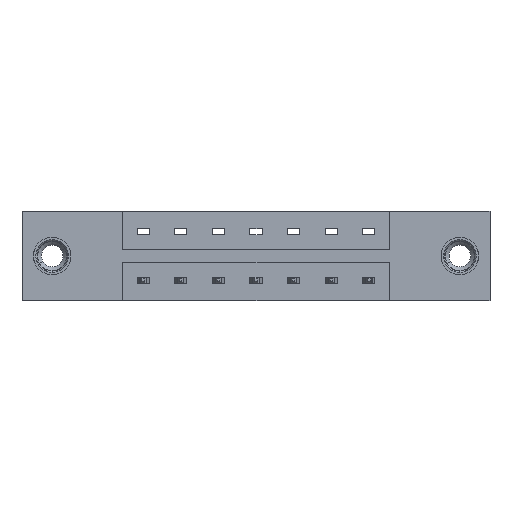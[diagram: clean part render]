
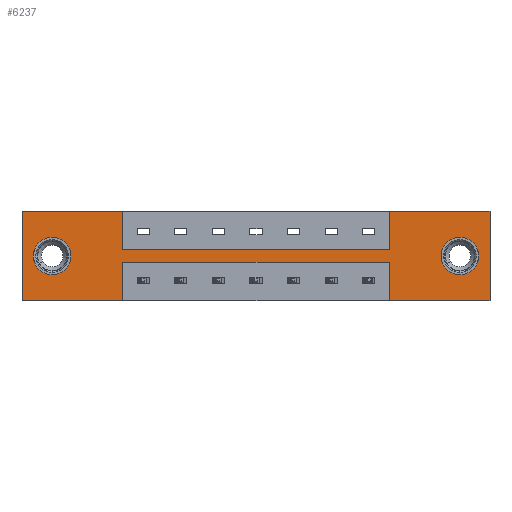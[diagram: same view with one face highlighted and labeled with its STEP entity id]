
A CAD part, front view. The second image highlights one B-rep face of the part: STEP entity #6237.
In plain terms, the highlighted planar face has unit normal (0, -1, 0).
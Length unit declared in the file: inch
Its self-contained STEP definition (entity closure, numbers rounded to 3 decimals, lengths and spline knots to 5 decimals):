
#14 = CARTESIAN_POINT ( 'NONE',  ( 0., 0., -0.37 ) ) ;
#27 = DIRECTION ( 'NONE',  ( 0., 0., 1. ) ) ;
#62 = DIRECTION ( 'NONE',  ( -1., 0., 0. ) ) ;
#170 = CARTESIAN_POINT ( 'NONE',  ( 0.4175, 0., -0.1585 ) ) ;
#188 = CARTESIAN_POINT ( 'NONE',  ( 1.815, 0., -0.107 ) ) ;
#285 = AXIS2_PLACEMENT_3D ( 'NONE', #14, #2483, #7926 ) ;
#487 = DIRECTION ( 'NONE',  ( 0., 0., 1. ) ) ;
#496 = DIRECTION ( 'NONE',  ( 0., 1., 0. ) ) ;
#583 = CARTESIAN_POINT ( 'NONE',  ( 1.5225, 0., -0.37 ) ) ;
#761 = DIRECTION ( 'NONE',  ( 1., 0., 0. ) ) ;
#781 = LINE ( 'NONE', #9023, #4622 ) ;
#893 = DIRECTION ( 'NONE',  ( 0., 0., 1. ) ) ;
#944 = EDGE_CURVE ( 'NONE', #3710, #7768, #3783, .T. ) ;
#968 = VERTEX_POINT ( 'NONE', #1865 ) ;
#1008 = CIRCLE ( 'NONE', #4218, 0.078 ) ;
#1221 = EDGE_CURVE ( 'NONE', #5632, #3437, #3912, .T. ) ;
#1270 = EDGE_LOOP ( 'NONE', ( #5932, #6631 ) ) ;
#1351 = EDGE_CURVE ( 'NONE', #3437, #5632, #5506, .T. ) ;
#1392 = LINE ( 'NONE', #2185, #3316 ) ;
#1398 = VECTOR ( 'NONE', #5048, 39.37008 ) ;
#1605 = VECTOR ( 'NONE', #6595, 39.37008 ) ;
#1644 = LINE ( 'NONE', #6472, #9361 ) ;
#1843 = DIRECTION ( 'NONE',  ( 0., 0., -1. ) ) ;
#1865 = CARTESIAN_POINT ( 'NONE',  ( 0.4175, 0., 0. ) ) ;
#1885 = ORIENTED_EDGE ( 'NONE', *, *, #6603, .F. ) ;
#1977 = VECTOR ( 'NONE', #4040, 39.37008 ) ;
#2023 = VERTEX_POINT ( 'NONE', #8441 ) ;
#2123 = EDGE_CURVE ( 'NONE', #9474, #9838, #4130, .T. ) ;
#2182 = ORIENTED_EDGE ( 'NONE', *, *, #6056, .F. ) ;
#2185 = CARTESIAN_POINT ( 'NONE',  ( 0.4175, 0., -0.2115 ) ) ;
#2227 = LINE ( 'NONE', #6493, #6210 ) ;
#2298 = CARTESIAN_POINT ( 'NONE',  ( 1.815, 0., -0.185 ) ) ;
#2483 = DIRECTION ( 'NONE',  ( 0., -1., 0. ) ) ;
#2548 = ORIENTED_EDGE ( 'NONE', *, *, #9210, .F. ) ;
#2790 = EDGE_CURVE ( 'NONE', #4205, #4442, #7013, .T. ) ;
#2955 = CIRCLE ( 'NONE', #7912, 0.078 ) ;
#2997 = AXIS2_PLACEMENT_3D ( 'NONE', #2298, #7767, #3133 ) ;
#3133 = DIRECTION ( 'NONE',  ( 0., 0., -1. ) ) ;
#3269 = ORIENTED_EDGE ( 'NONE', *, *, #8101, .F. ) ;
#3316 = VECTOR ( 'NONE', #6151, 39.37008 ) ;
#3437 = VERTEX_POINT ( 'NONE', #188 ) ;
#3454 = EDGE_LOOP ( 'NONE', ( #8373, #5009, #7488, #7731, #4653, #7401, #4663, #3269, #1885, #6809, #2182, #2548 ) ) ;
#3586 = LINE ( 'NONE', #170, #1398 ) ;
#3659 = CARTESIAN_POINT ( 'NONE',  ( 0.125, 0., -0.185 ) ) ;
#3710 = VERTEX_POINT ( 'NONE', #9767 ) ;
#3752 = VECTOR ( 'NONE', #1843, 39.37008 ) ;
#3783 = LINE ( 'NONE', #4272, #1605 ) ;
#3912 = CIRCLE ( 'NONE', #9789, 0.078 ) ;
#3968 = VERTEX_POINT ( 'NONE', #6441 ) ;
#4040 = DIRECTION ( 'NONE',  ( 1., 0., 0. ) ) ;
#4127 = FACE_BOUND ( 'NONE', #9664, .T. ) ;
#4130 = LINE ( 'NONE', #7097, #1977 ) ;
#4162 = DIRECTION ( 'NONE',  ( 0., 0., -1. ) ) ;
#4205 = VERTEX_POINT ( 'NONE', #7428 ) ;
#4218 = AXIS2_PLACEMENT_3D ( 'NONE', #3659, #8965, #4473 ) ;
#4272 = CARTESIAN_POINT ( 'NONE',  ( 0., 0., -0.37 ) ) ;
#4442 = VERTEX_POINT ( 'NONE', #583 ) ;
#4473 = DIRECTION ( 'NONE',  ( 0., 0., 1. ) ) ;
#4622 = VECTOR ( 'NONE', #487, 39.37008 ) ;
#4647 = VERTEX_POINT ( 'NONE', #7895 ) ;
#4653 = ORIENTED_EDGE ( 'NONE', *, *, #5365, .F. ) ;
#4663 = ORIENTED_EDGE ( 'NONE', *, *, #7560, .F. ) ;
#4750 = VECTOR ( 'NONE', #62, 39.37008 ) ;
#4771 = CARTESIAN_POINT ( 'NONE',  ( 1.94, 0., 0. ) ) ;
#4911 = DIRECTION ( 'NONE',  ( 0., 1., 0. ) ) ;
#5009 = ORIENTED_EDGE ( 'NONE', *, *, #2790, .F. ) ;
#5048 = DIRECTION ( 'NONE',  ( 0., 0., -1. ) ) ;
#5213 = LINE ( 'NONE', #10012, #6735 ) ;
#5365 = EDGE_CURVE ( 'NONE', #9838, #9580, #2227, .T. ) ;
#5372 = CARTESIAN_POINT ( 'NONE',  ( 1.815, 0., -0.185 ) ) ;
#5506 = CIRCLE ( 'NONE', #2997, 0.078 ) ;
#5632 = VERTEX_POINT ( 'NONE', #6089 ) ;
#5721 = CARTESIAN_POINT ( 'NONE',  ( 0., 0., -0.37 ) ) ;
#5821 = VECTOR ( 'NONE', #6305, 39.37008 ) ;
#5841 = CARTESIAN_POINT ( 'NONE',  ( 0., 0., 0. ) ) ;
#5914 = DIRECTION ( 'NONE',  ( 0., 0., 1. ) ) ;
#5932 = ORIENTED_EDGE ( 'NONE', *, *, #1351, .T. ) ;
#5948 = ORIENTED_EDGE ( 'NONE', *, *, #9083, .T. ) ;
#6056 = EDGE_CURVE ( 'NONE', #3968, #3710, #9971, .T. ) ;
#6089 = CARTESIAN_POINT ( 'NONE',  ( 1.815, 0., -0.263 ) ) ;
#6128 = DIRECTION ( 'NONE',  ( 0., 0., -1. ) ) ;
#6151 = DIRECTION ( 'NONE',  ( -1., 0., 0. ) ) ;
#6210 = VECTOR ( 'NONE', #893, 39.37008 ) ;
#6237 = ADVANCED_FACE ( 'NONE', ( #7946, #4127, #6430 ), #7183, .T. ) ;
#6305 = DIRECTION ( 'NONE',  ( 1., 0., 0. ) ) ;
#6430 = FACE_OUTER_BOUND ( 'NONE', #3454, .T. ) ;
#6441 = CARTESIAN_POINT ( 'NONE',  ( 0.4175, 0., -0.2115 ) ) ;
#6472 = CARTESIAN_POINT ( 'NONE',  ( 1.94, 0., 0. ) ) ;
#6493 = CARTESIAN_POINT ( 'NONE',  ( 1.5225, 0., -0.1585 ) ) ;
#6595 = DIRECTION ( 'NONE',  ( -1., 0., 0. ) ) ;
#6603 = EDGE_CURVE ( 'NONE', #7768, #8918, #781, .T. ) ;
#6631 = ORIENTED_EDGE ( 'NONE', *, *, #1221, .T. ) ;
#6682 = CARTESIAN_POINT ( 'NONE',  ( 0., 0., -0.37 ) ) ;
#6735 = VECTOR ( 'NONE', #761, 39.37008 ) ;
#6809 = ORIENTED_EDGE ( 'NONE', *, *, #944, .F. ) ;
#7013 = LINE ( 'NONE', #5721, #4750 ) ;
#7097 = CARTESIAN_POINT ( 'NONE',  ( 0.4175, 0., -0.1585 ) ) ;
#7183 = PLANE ( 'NONE',  #285 ) ;
#7244 = CARTESIAN_POINT ( 'NONE',  ( 0.4175, 0., -0.1585 ) ) ;
#7318 = EDGE_CURVE ( 'NONE', #9580, #8051, #8253, .T. ) ;
#7401 = ORIENTED_EDGE ( 'NONE', *, *, #2123, .F. ) ;
#7428 = CARTESIAN_POINT ( 'NONE',  ( 1.94, 0., -0.37 ) ) ;
#7432 = EDGE_CURVE ( 'NONE', #4647, #2023, #2955, .T. ) ;
#7488 = ORIENTED_EDGE ( 'NONE', *, *, #10019, .F. ) ;
#7547 = VERTEX_POINT ( 'NONE', #8745 ) ;
#7560 = EDGE_CURVE ( 'NONE', #968, #9474, #3586, .T. ) ;
#7731 = ORIENTED_EDGE ( 'NONE', *, *, #7318, .F. ) ;
#7767 = DIRECTION ( 'NONE',  ( 0., 1., 0. ) ) ;
#7768 = VERTEX_POINT ( 'NONE', #6682 ) ;
#7895 = CARTESIAN_POINT ( 'NONE',  ( 0.125, 0., -0.107 ) ) ;
#7912 = AXIS2_PLACEMENT_3D ( 'NONE', #9359, #4911, #27 ) ;
#7926 = DIRECTION ( 'NONE',  ( 0., 0., -1. ) ) ;
#7931 = VECTOR ( 'NONE', #5914, 39.37008 ) ;
#7946 = FACE_BOUND ( 'NONE', #1270, .T. ) ;
#8051 = VERTEX_POINT ( 'NONE', #4771 ) ;
#8101 = EDGE_CURVE ( 'NONE', #8918, #968, #5213, .T. ) ;
#8150 = LINE ( 'NONE', #9576, #7931 ) ;
#8160 = CARTESIAN_POINT ( 'NONE',  ( 1.5225, 0., 0. ) ) ;
#8253 = LINE ( 'NONE', #9948, #5821 ) ;
#8350 = EDGE_CURVE ( 'NONE', #4442, #7547, #8150, .T. ) ;
#8373 = ORIENTED_EDGE ( 'NONE', *, *, #8350, .F. ) ;
#8441 = CARTESIAN_POINT ( 'NONE',  ( 0.125, 0., -0.263 ) ) ;
#8745 = CARTESIAN_POINT ( 'NONE',  ( 1.5225, 0., -0.2115 ) ) ;
#8755 = CARTESIAN_POINT ( 'NONE',  ( 0.4175, 0., -0.2115 ) ) ;
#8918 = VERTEX_POINT ( 'NONE', #5841 ) ;
#8944 = ORIENTED_EDGE ( 'NONE', *, *, #7432, .T. ) ;
#8965 = DIRECTION ( 'NONE',  ( 0., 1., 0. ) ) ;
#9023 = CARTESIAN_POINT ( 'NONE',  ( 0., 0., 0. ) ) ;
#9083 = EDGE_CURVE ( 'NONE', #2023, #4647, #1008, .T. ) ;
#9174 = CARTESIAN_POINT ( 'NONE',  ( 1.5225, 0., -0.1585 ) ) ;
#9210 = EDGE_CURVE ( 'NONE', #7547, #3968, #1392, .T. ) ;
#9359 = CARTESIAN_POINT ( 'NONE',  ( 0.125, 0., -0.185 ) ) ;
#9361 = VECTOR ( 'NONE', #4162, 39.37008 ) ;
#9474 = VERTEX_POINT ( 'NONE', #7244 ) ;
#9576 = CARTESIAN_POINT ( 'NONE',  ( 1.5225, 0., -0.2115 ) ) ;
#9580 = VERTEX_POINT ( 'NONE', #8160 ) ;
#9664 = EDGE_LOOP ( 'NONE', ( #8944, #5948 ) ) ;
#9767 = CARTESIAN_POINT ( 'NONE',  ( 0.4175, 0., -0.37 ) ) ;
#9789 = AXIS2_PLACEMENT_3D ( 'NONE', #5372, #496, #6128 ) ;
#9838 = VERTEX_POINT ( 'NONE', #9174 ) ;
#9948 = CARTESIAN_POINT ( 'NONE',  ( 0., 0., 0. ) ) ;
#9971 = LINE ( 'NONE', #8755, #3752 ) ;
#10012 = CARTESIAN_POINT ( 'NONE',  ( 0., 0., 0. ) ) ;
#10019 = EDGE_CURVE ( 'NONE', #8051, #4205, #1644, .T. ) ;
